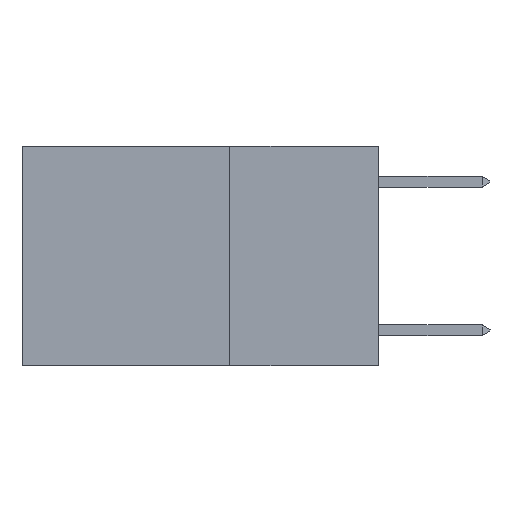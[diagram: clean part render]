
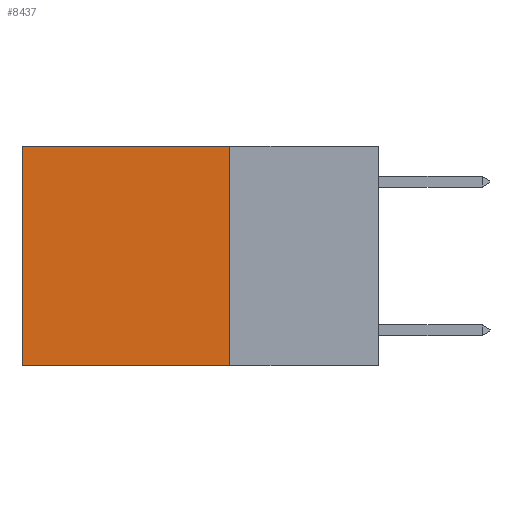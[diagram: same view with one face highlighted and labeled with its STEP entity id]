
A CAD part, left-side view. The second image highlights one B-rep face of the part: STEP entity #8437.
In plain terms, the highlighted planar face has unit normal (-1, 0, 0).
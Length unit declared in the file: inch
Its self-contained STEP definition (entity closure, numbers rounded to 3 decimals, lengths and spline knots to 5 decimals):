
#510 = EDGE_CURVE ( 'NONE', #656, #18254, #8719, .T. ) ;
#656 = VERTEX_POINT ( 'NONE', #4753 ) ;
#789 = VERTEX_POINT ( 'NONE', #3573 ) ;
#834 = DIRECTION ( 'NONE',  ( 0., 1., 0. ) ) ;
#1074 = ORIENTED_EDGE ( 'NONE', *, *, #510, .T. ) ;
#1192 = VECTOR ( 'NONE', #834, 39.37008 ) ;
#1541 = CARTESIAN_POINT ( 'NONE',  ( 0.2625, 0.25, -0.37 ) ) ;
#2569 = EDGE_CURVE ( 'NONE', #789, #12429, #3552, .T. ) ;
#2582 = PLANE ( 'NONE',  #5373 ) ;
#3552 = LINE ( 'NONE', #15020, #7058 ) ;
#3573 = CARTESIAN_POINT ( 'NONE',  ( 0.2625, 0.25, 0. ) ) ;
#4753 = CARTESIAN_POINT ( 'NONE',  ( 0.2625, 0.6, 0. ) ) ;
#4870 = CARTESIAN_POINT ( 'NONE',  ( 0.2625, 0.25, -0.37 ) ) ;
#5169 = LINE ( 'NONE', #18650, #1192 ) ;
#5373 = AXIS2_PLACEMENT_3D ( 'NONE', #5555, #7060, #5486 ) ;
#5486 = DIRECTION ( 'NONE',  ( 0., 0., -1. ) ) ;
#5555 = CARTESIAN_POINT ( 'NONE',  ( 0.2625, 0.25, 0. ) ) ;
#7058 = VECTOR ( 'NONE', #9062, 39.37008 ) ;
#7060 = DIRECTION ( 'NONE',  ( 1., 0., 0. ) ) ;
#7307 = DIRECTION ( 'NONE',  ( 0., 0., -1. ) ) ;
#8437 = ADVANCED_FACE ( 'NONE', ( #12888 ), #2582, .F. ) ;
#8719 = LINE ( 'NONE', #16180, #9178 ) ;
#9024 = DIRECTION ( 'NONE',  ( 0., 1., 0. ) ) ;
#9041 = ORIENTED_EDGE ( 'NONE', *, *, #15830, .F. ) ;
#9060 = EDGE_LOOP ( 'NONE', ( #1074, #9041, #11750, #11354 ) ) ;
#9062 = DIRECTION ( 'NONE',  ( 0., 0., -1. ) ) ;
#9178 = VECTOR ( 'NONE', #7307, 39.37008 ) ;
#9886 = VECTOR ( 'NONE', #9024, 39.37008 ) ;
#10054 = EDGE_CURVE ( 'NONE', #789, #656, #5169, .T. ) ;
#11354 = ORIENTED_EDGE ( 'NONE', *, *, #10054, .T. ) ;
#11750 = ORIENTED_EDGE ( 'NONE', *, *, #2569, .F. ) ;
#12429 = VERTEX_POINT ( 'NONE', #4870 ) ;
#12888 = FACE_OUTER_BOUND ( 'NONE', #9060, .T. ) ;
#13809 = LINE ( 'NONE', #1541, #9886 ) ;
#15020 = CARTESIAN_POINT ( 'NONE',  ( 0.2625, 0.25, 0. ) ) ;
#15217 = CARTESIAN_POINT ( 'NONE',  ( 0.2625, 0.6, -0.37 ) ) ;
#15830 = EDGE_CURVE ( 'NONE', #12429, #18254, #13809, .T. ) ;
#16180 = CARTESIAN_POINT ( 'NONE',  ( 0.2625, 0.6, 0. ) ) ;
#18254 = VERTEX_POINT ( 'NONE', #15217 ) ;
#18650 = CARTESIAN_POINT ( 'NONE',  ( 0.2625, 0.25, 0. ) ) ;
